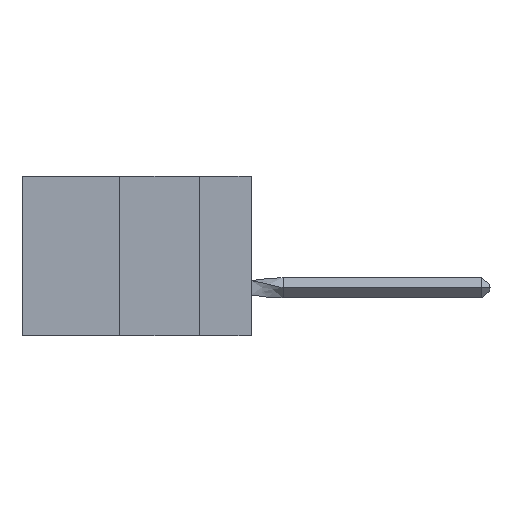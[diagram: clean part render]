
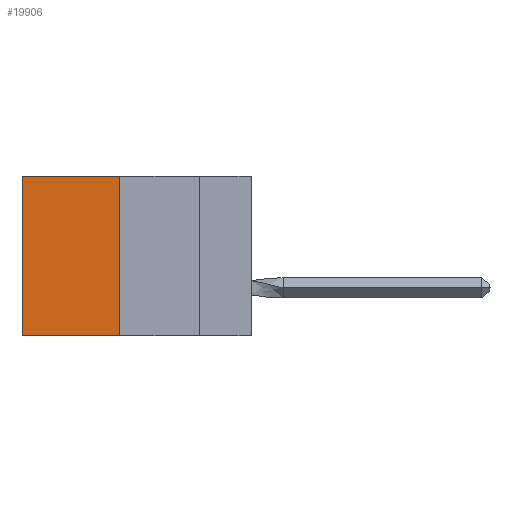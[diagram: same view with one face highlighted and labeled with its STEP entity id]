
A CAD part, left-side view. The second image highlights one B-rep face of the part: STEP entity #19906.
In plain terms, the highlighted planar face has unit normal (-1, 0, 0).
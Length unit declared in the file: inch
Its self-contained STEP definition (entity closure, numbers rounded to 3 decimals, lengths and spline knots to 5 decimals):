
#25 = CARTESIAN_POINT ( 'NONE',  ( 0.305, 0.413, -0.5 ) ) ;
#271 = VERTEX_POINT ( 'NONE', #18368 ) ;
#470 = PLANE ( 'NONE',  #17061 ) ;
#1034 = VECTOR ( 'NONE', #4158, 39.37008 ) ;
#1157 = VECTOR ( 'NONE', #3849, 39.37008 ) ;
#1255 = VECTOR ( 'NONE', #19495, 39.37008 ) ;
#3152 = EDGE_LOOP ( 'NONE', ( #16177, #16099, #11032, #21234 ) ) ;
#3340 = EDGE_CURVE ( 'NONE', #21216, #22759, #13411, .T. ) ;
#3849 = DIRECTION ( 'NONE',  ( 0., 0., -1. ) ) ;
#4059 = FACE_OUTER_BOUND ( 'NONE', #3152, .T. ) ;
#4158 = DIRECTION ( 'NONE',  ( 0., 1., 0. ) ) ;
#4391 = LINE ( 'NONE', #8229, #18618 ) ;
#4586 = CARTESIAN_POINT ( 'NONE',  ( 0.305, 0.413, 0. ) ) ;
#5987 = EDGE_CURVE ( 'NONE', #21731, #271, #9094, .T. ) ;
#6228 = CARTESIAN_POINT ( 'NONE',  ( 0.305, 0.72, 0. ) ) ;
#8229 = CARTESIAN_POINT ( 'NONE',  ( 0.305, 0.413, -0.5 ) ) ;
#9094 = LINE ( 'NONE', #25, #1157 ) ;
#9963 = CARTESIAN_POINT ( 'NONE',  ( 0.305, 0.413, 0. ) ) ;
#11032 = ORIENTED_EDGE ( 'NONE', *, *, #5987, .F. ) ;
#11091 = LINE ( 'NONE', #9963, #1034 ) ;
#11797 = EDGE_CURVE ( 'NONE', #271, #22759, #4391, .T. ) ;
#13411 = LINE ( 'NONE', #21544, #1255 ) ;
#14025 = DIRECTION ( 'NONE',  ( 0., 1., 0. ) ) ;
#16099 = ORIENTED_EDGE ( 'NONE', *, *, #11797, .F. ) ;
#16161 = DIRECTION ( 'NONE',  ( 1., 0., 0. ) ) ;
#16177 = ORIENTED_EDGE ( 'NONE', *, *, #3340, .T. ) ;
#17061 = AXIS2_PLACEMENT_3D ( 'NONE', #22109, #16161, #21850 ) ;
#18006 = CARTESIAN_POINT ( 'NONE',  ( 0.305, 0.72, -0.5 ) ) ;
#18368 = CARTESIAN_POINT ( 'NONE',  ( 0.305, 0.413, -0.5 ) ) ;
#18618 = VECTOR ( 'NONE', #14025, 39.37008 ) ;
#19351 = EDGE_CURVE ( 'NONE', #21731, #21216, #11091, .T. ) ;
#19495 = DIRECTION ( 'NONE',  ( 0., 0., -1. ) ) ;
#19906 = ADVANCED_FACE ( 'NONE', ( #4059 ), #470, .F. ) ;
#21216 = VERTEX_POINT ( 'NONE', #6228 ) ;
#21234 = ORIENTED_EDGE ( 'NONE', *, *, #19351, .T. ) ;
#21544 = CARTESIAN_POINT ( 'NONE',  ( 0.305, 0.72, -0.5 ) ) ;
#21731 = VERTEX_POINT ( 'NONE', #4586 ) ;
#21850 = DIRECTION ( 'NONE',  ( 0., 0., -1. ) ) ;
#22109 = CARTESIAN_POINT ( 'NONE',  ( 0.305, 0.413, -0.5 ) ) ;
#22759 = VERTEX_POINT ( 'NONE', #18006 ) ;
